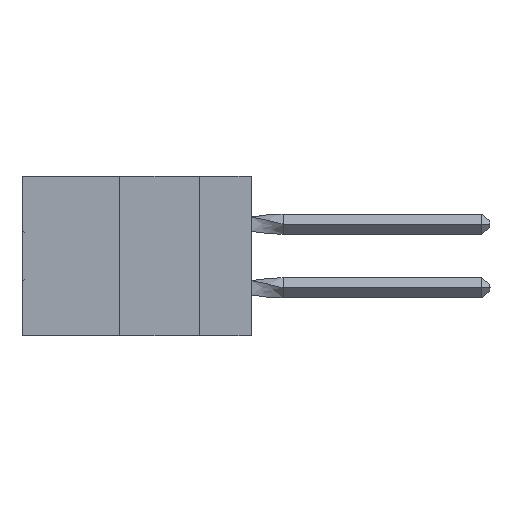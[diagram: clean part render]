
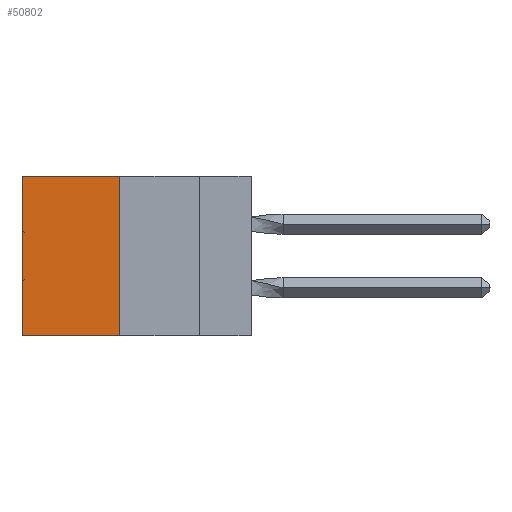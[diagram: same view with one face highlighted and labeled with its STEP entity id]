
A CAD part, left-side view. The second image highlights one B-rep face of the part: STEP entity #50802.
In plain terms, the highlighted planar face has unit normal (-1, 0, 0).
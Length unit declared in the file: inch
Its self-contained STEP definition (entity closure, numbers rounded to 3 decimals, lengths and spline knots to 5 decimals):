
#481 = EDGE_CURVE ( 'NONE', #30712, #42731, #12862, .T. ) ;
#485 = DIRECTION ( 'NONE',  ( 1., 0., 0. ) ) ;
#1326 = LINE ( 'NONE', #3826, #53427 ) ;
#3282 = DIRECTION ( 'NONE',  ( 0., 1., 0. ) ) ;
#3826 = CARTESIAN_POINT ( 'NONE',  ( 0.305, 0.413, 0. ) ) ;
#4593 = DIRECTION ( 'NONE',  ( 0., 0., -1. ) ) ;
#8032 = LINE ( 'NONE', #52762, #15329 ) ;
#9524 = CARTESIAN_POINT ( 'NONE',  ( 0.305, 0.72, -0.5 ) ) ;
#12862 = LINE ( 'NONE', #9524, #54299 ) ;
#13993 = CARTESIAN_POINT ( 'NONE',  ( 0.305, 0.413, -0.5 ) ) ;
#14167 = VERTEX_POINT ( 'NONE', #13993 ) ;
#15329 = VECTOR ( 'NONE', #48294, 39.37008 ) ;
#18339 = EDGE_CURVE ( 'NONE', #27496, #14167, #8032, .T. ) ;
#18367 = AXIS2_PLACEMENT_3D ( 'NONE', #51823, #485, #4593 ) ;
#19672 = ORIENTED_EDGE ( 'NONE', *, *, #32976, .T. ) ;
#25644 = VECTOR ( 'NONE', #47517, 39.37008 ) ;
#27496 = VERTEX_POINT ( 'NONE', #37915 ) ;
#27593 = ORIENTED_EDGE ( 'NONE', *, *, #481, .T. ) ;
#27766 = EDGE_CURVE ( 'NONE', #14167, #42731, #43703, .T. ) ;
#29088 = EDGE_LOOP ( 'NONE', ( #27593, #43908, #45795, #19672 ) ) ;
#30712 = VERTEX_POINT ( 'NONE', #42577 ) ;
#32976 = EDGE_CURVE ( 'NONE', #27496, #30712, #1326, .T. ) ;
#37915 = CARTESIAN_POINT ( 'NONE',  ( 0.305, 0.413, 0. ) ) ;
#42577 = CARTESIAN_POINT ( 'NONE',  ( 0.305, 0.72, 0. ) ) ;
#42731 = VERTEX_POINT ( 'NONE', #48065 ) ;
#43703 = LINE ( 'NONE', #52187, #25644 ) ;
#43908 = ORIENTED_EDGE ( 'NONE', *, *, #27766, .F. ) ;
#45145 = FACE_OUTER_BOUND ( 'NONE', #29088, .T. ) ;
#45795 = ORIENTED_EDGE ( 'NONE', *, *, #18339, .F. ) ;
#47517 = DIRECTION ( 'NONE',  ( 0., 1., 0. ) ) ;
#47765 = DIRECTION ( 'NONE',  ( 0., 0., -1. ) ) ;
#48065 = CARTESIAN_POINT ( 'NONE',  ( 0.305, 0.72, -0.5 ) ) ;
#48294 = DIRECTION ( 'NONE',  ( 0., 0., -1. ) ) ;
#50802 = ADVANCED_FACE ( 'NONE', ( #45145 ), #51635, .F. ) ;
#51635 = PLANE ( 'NONE',  #18367 ) ;
#51823 = CARTESIAN_POINT ( 'NONE',  ( 0.305, 0.413, -0.5 ) ) ;
#52187 = CARTESIAN_POINT ( 'NONE',  ( 0.305, 0.413, -0.5 ) ) ;
#52762 = CARTESIAN_POINT ( 'NONE',  ( 0.305, 0.413, -0.5 ) ) ;
#53427 = VECTOR ( 'NONE', #3282, 39.37008 ) ;
#54299 = VECTOR ( 'NONE', #47765, 39.37008 ) ;
